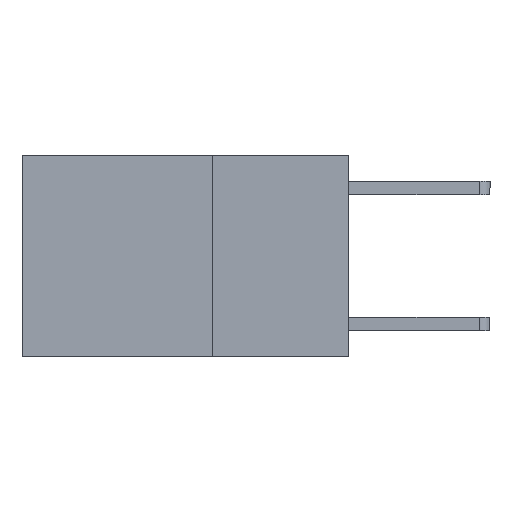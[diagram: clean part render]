
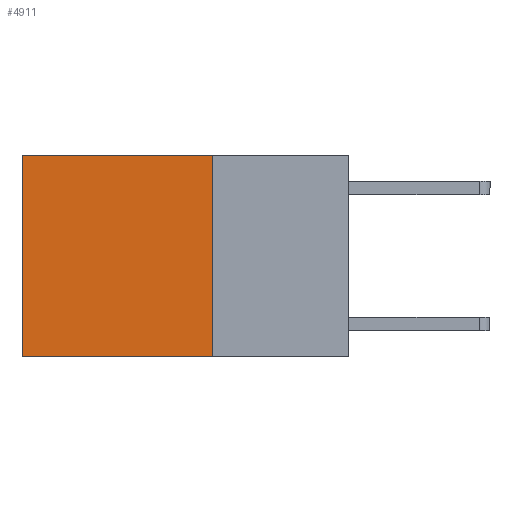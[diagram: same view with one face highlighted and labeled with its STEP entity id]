
A CAD part, left-side view. The second image highlights one B-rep face of the part: STEP entity #4911.
In plain terms, the highlighted planar face has unit normal (-1, 0, 0).
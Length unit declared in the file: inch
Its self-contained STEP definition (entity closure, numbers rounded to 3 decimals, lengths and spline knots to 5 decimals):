
#217 = PLANE ( 'NONE',  #9684 ) ;
#317 = ORIENTED_EDGE ( 'NONE', *, *, #372, .F. ) ;
#372 = EDGE_CURVE ( 'NONE', #4460, #9213, #3611, .T. ) ;
#535 = CARTESIAN_POINT ( 'NONE',  ( 0.2625, 0.25, 0. ) ) ;
#1093 = LINE ( 'NONE', #3405, #9514 ) ;
#1192 = VERTEX_POINT ( 'NONE', #10120 ) ;
#1196 = CARTESIAN_POINT ( 'NONE',  ( 0.2625, 0.25, -0.37 ) ) ;
#1304 = VERTEX_POINT ( 'NONE', #6241 ) ;
#1391 = LINE ( 'NONE', #1196, #8226 ) ;
#1574 = DIRECTION ( 'NONE',  ( 0., 0., -1. ) ) ;
#2143 = CARTESIAN_POINT ( 'NONE',  ( 0.2625, 0.25, 0. ) ) ;
#3230 = ORIENTED_EDGE ( 'NONE', *, *, #10241, .T. ) ;
#3404 = ORIENTED_EDGE ( 'NONE', *, *, #5134, .T. ) ;
#3405 = CARTESIAN_POINT ( 'NONE',  ( 0.2625, 0.6, 0. ) ) ;
#3459 = EDGE_LOOP ( 'NONE', ( #3404, #8163, #317, #3230 ) ) ;
#3611 = LINE ( 'NONE', #2143, #3618 ) ;
#3618 = VECTOR ( 'NONE', #4562, 39.37008 ) ;
#4460 = VERTEX_POINT ( 'NONE', #535 ) ;
#4562 = DIRECTION ( 'NONE',  ( 0., 0., -1. ) ) ;
#4630 = CARTESIAN_POINT ( 'NONE',  ( 0.2625, 0.25, 0. ) ) ;
#4770 = DIRECTION ( 'NONE',  ( 1., 0., 0. ) ) ;
#4911 = ADVANCED_FACE ( 'NONE', ( #8388 ), #217, .F. ) ;
#5134 = EDGE_CURVE ( 'NONE', #1304, #1192, #1093, .T. ) ;
#5431 = LINE ( 'NONE', #4630, #10224 ) ;
#6241 = CARTESIAN_POINT ( 'NONE',  ( 0.2625, 0.6, 0. ) ) ;
#6632 = DIRECTION ( 'NONE',  ( 0., 0., -1. ) ) ;
#6908 = CARTESIAN_POINT ( 'NONE',  ( 0.2625, 0.25, -0.37 ) ) ;
#6932 = DIRECTION ( 'NONE',  ( 0., 1., 0. ) ) ;
#7107 = CARTESIAN_POINT ( 'NONE',  ( 0.2625, 0.25, 0. ) ) ;
#8163 = ORIENTED_EDGE ( 'NONE', *, *, #9761, .F. ) ;
#8226 = VECTOR ( 'NONE', #6932, 39.37008 ) ;
#8388 = FACE_OUTER_BOUND ( 'NONE', #3459, .T. ) ;
#9213 = VERTEX_POINT ( 'NONE', #6908 ) ;
#9426 = DIRECTION ( 'NONE',  ( 0., 1., 0. ) ) ;
#9514 = VECTOR ( 'NONE', #6632, 39.37008 ) ;
#9684 = AXIS2_PLACEMENT_3D ( 'NONE', #7107, #4770, #1574 ) ;
#9761 = EDGE_CURVE ( 'NONE', #9213, #1192, #1391, .T. ) ;
#10120 = CARTESIAN_POINT ( 'NONE',  ( 0.2625, 0.6, -0.37 ) ) ;
#10224 = VECTOR ( 'NONE', #9426, 39.37008 ) ;
#10241 = EDGE_CURVE ( 'NONE', #4460, #1304, #5431, .T. ) ;
